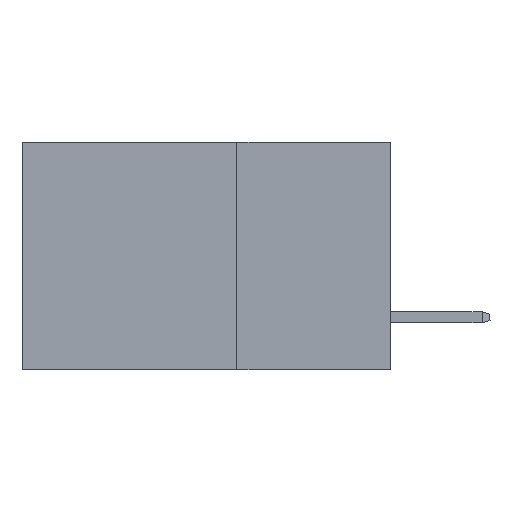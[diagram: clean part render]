
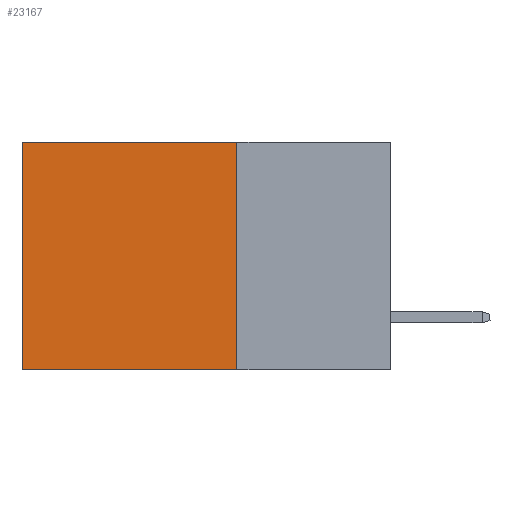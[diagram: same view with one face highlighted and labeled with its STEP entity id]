
A CAD part, left-side view. The second image highlights one B-rep face of the part: STEP entity #23167.
In plain terms, the highlighted planar face has unit normal (-1, 0, 0).
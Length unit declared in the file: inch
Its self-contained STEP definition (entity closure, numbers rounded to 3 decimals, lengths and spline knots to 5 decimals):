
#129 = CARTESIAN_POINT ( 'NONE',  ( 0.2875, 0.25, 0. ) ) ;
#1718 = DIRECTION ( 'NONE',  ( 0., 0., -1. ) ) ;
#2118 = CARTESIAN_POINT ( 'NONE',  ( 0.2875, 0.6, -0.37 ) ) ;
#2286 = EDGE_CURVE ( 'NONE', #17330, #4765, #20433, .T. ) ;
#2584 = FACE_OUTER_BOUND ( 'NONE', #17948, .T. ) ;
#2773 = ORIENTED_EDGE ( 'NONE', *, *, #18579, .T. ) ;
#3283 = VECTOR ( 'NONE', #15048, 39.37008 ) ;
#3497 = VECTOR ( 'NONE', #15279, 39.37008 ) ;
#3940 = ORIENTED_EDGE ( 'NONE', *, *, #19146, .T. ) ;
#4139 = CARTESIAN_POINT ( 'NONE',  ( 0.2875, 0.25, -0.37 ) ) ;
#4765 = VERTEX_POINT ( 'NONE', #4139 ) ;
#5326 = CARTESIAN_POINT ( 'NONE',  ( 0.2875, 0.25, 0. ) ) ;
#6002 = VECTOR ( 'NONE', #9254, 39.37008 ) ;
#6142 = ORIENTED_EDGE ( 'NONE', *, *, #2286, .F. ) ;
#6612 = LINE ( 'NONE', #5326, #6002 ) ;
#9107 = LINE ( 'NONE', #22819, #3283 ) ;
#9254 = DIRECTION ( 'NONE',  ( 0., 1., 0. ) ) ;
#9999 = AXIS2_PLACEMENT_3D ( 'NONE', #25202, #13487, #1718 ) ;
#10030 = CARTESIAN_POINT ( 'NONE',  ( 0.2875, 0.6, 0. ) ) ;
#11522 = PLANE ( 'NONE',  #9999 ) ;
#11956 = DIRECTION ( 'NONE',  ( 0., 0., -1. ) ) ;
#13487 = DIRECTION ( 'NONE',  ( 1., 0., 0. ) ) ;
#15048 = DIRECTION ( 'NONE',  ( 0., 0., -1. ) ) ;
#15279 = DIRECTION ( 'NONE',  ( 0., 1., 0. ) ) ;
#17261 = CARTESIAN_POINT ( 'NONE',  ( 0.2875, 0.25, -0.37 ) ) ;
#17330 = VERTEX_POINT ( 'NONE', #23729 ) ;
#17948 = EDGE_LOOP ( 'NONE', ( #2773, #22021, #6142, #3940 ) ) ;
#18579 = EDGE_CURVE ( 'NONE', #23330, #22001, #9107, .T. ) ;
#19146 = EDGE_CURVE ( 'NONE', #17330, #23330, #6612, .T. ) ;
#19221 = VECTOR ( 'NONE', #11956, 39.37008 ) ;
#20433 = LINE ( 'NONE', #129, #19221 ) ;
#22001 = VERTEX_POINT ( 'NONE', #2118 ) ;
#22021 = ORIENTED_EDGE ( 'NONE', *, *, #23789, .F. ) ;
#22819 = CARTESIAN_POINT ( 'NONE',  ( 0.2875, 0.6, 0. ) ) ;
#23167 = ADVANCED_FACE ( 'NONE', ( #2584 ), #11522, .F. ) ;
#23330 = VERTEX_POINT ( 'NONE', #10030 ) ;
#23719 = LINE ( 'NONE', #17261, #3497 ) ;
#23729 = CARTESIAN_POINT ( 'NONE',  ( 0.2875, 0.25, 0. ) ) ;
#23789 = EDGE_CURVE ( 'NONE', #4765, #22001, #23719, .T. ) ;
#25202 = CARTESIAN_POINT ( 'NONE',  ( 0.2875, 0.25, 0. ) ) ;
